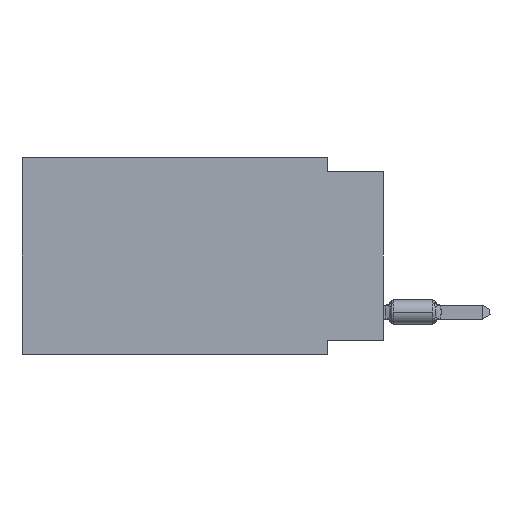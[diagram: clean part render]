
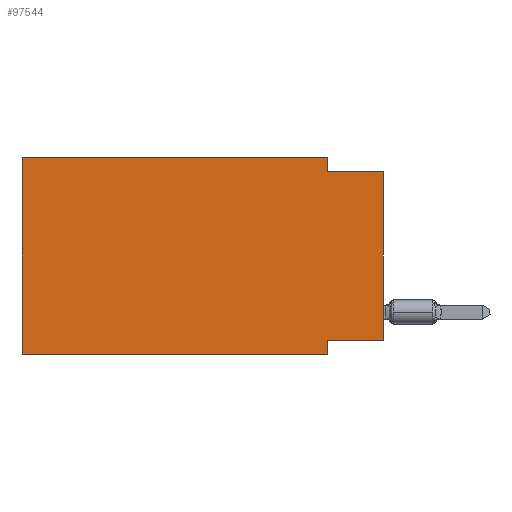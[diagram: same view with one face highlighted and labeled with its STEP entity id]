
A CAD part, left-side view. The second image highlights one B-rep face of the part: STEP entity #97544.
In plain terms, the highlighted planar face has unit normal (-1, 0, 0).
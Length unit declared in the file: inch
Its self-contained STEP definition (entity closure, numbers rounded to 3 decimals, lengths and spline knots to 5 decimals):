
#683 = PLANE ( 'NONE',  #84745 ) ;
#5026 = DIRECTION ( 'NONE',  ( 0., -1., 0. ) ) ;
#6773 = EDGE_CURVE ( 'NONE', #51343, #54908, #22327, .T. ) ;
#7010 = CARTESIAN_POINT ( 'NONE',  ( 0., 0.645, 0. ) ) ;
#9215 = VECTOR ( 'NONE', #25521, 39.37008 ) ;
#12195 = VERTEX_POINT ( 'NONE', #44199 ) ;
#14014 = CARTESIAN_POINT ( 'NONE',  ( 0., 0., -0.325 ) ) ;
#14069 = CARTESIAN_POINT ( 'NONE',  ( 0., 0.1, -0.325 ) ) ;
#15160 = FACE_OUTER_BOUND ( 'NONE', #84320, .T. ) ;
#15401 = LINE ( 'NONE', #47994, #83148 ) ;
#16739 = DIRECTION ( 'NONE',  ( 0., 0., 1. ) ) ;
#20035 = LINE ( 'NONE', #54736, #75508 ) ;
#21711 = CARTESIAN_POINT ( 'NONE',  ( 0., 0.1, -0.025 ) ) ;
#21777 = EDGE_CURVE ( 'NONE', #70939, #39694, #88263, .T. ) ;
#22327 = LINE ( 'NONE', #91770, #9215 ) ;
#23182 = DIRECTION ( 'NONE',  ( 0., 0., -1. ) ) ;
#24846 = ORIENTED_EDGE ( 'NONE', *, *, #70834, .T. ) ;
#25521 = DIRECTION ( 'NONE',  ( 0., -1., 0. ) ) ;
#28022 = CARTESIAN_POINT ( 'NONE',  ( 0., 0.1, 0. ) ) ;
#29117 = VECTOR ( 'NONE', #37099, 39.37008 ) ;
#32176 = DIRECTION ( 'NONE',  ( 0., 1., 0. ) ) ;
#33823 = DIRECTION ( 'NONE',  ( 1., 0., 0. ) ) ;
#34258 = LINE ( 'NONE', #73814, #103208 ) ;
#37099 = DIRECTION ( 'NONE',  ( 0., 0., -1. ) ) ;
#37621 = CARTESIAN_POINT ( 'NONE',  ( 0., 0.1, 0. ) ) ;
#39694 = VERTEX_POINT ( 'NONE', #7010 ) ;
#41822 = CARTESIAN_POINT ( 'NONE',  ( 0., 0.645, -0.35 ) ) ;
#44199 = CARTESIAN_POINT ( 'NONE',  ( 0., 0.1, -0.35 ) ) ;
#44645 = EDGE_CURVE ( 'NONE', #47113, #51343, #45103, .T. ) ;
#45103 = LINE ( 'NONE', #28022, #29117 ) ;
#46551 = DIRECTION ( 'NONE',  ( 0., 0., 1. ) ) ;
#47089 = EDGE_CURVE ( 'NONE', #70939, #12195, #20035, .T. ) ;
#47113 = VERTEX_POINT ( 'NONE', #37621 ) ;
#47994 = CARTESIAN_POINT ( 'NONE',  ( 0., 0.645, 0. ) ) ;
#49284 = ORIENTED_EDGE ( 'NONE', *, *, #6773, .F. ) ;
#50592 = ORIENTED_EDGE ( 'NONE', *, *, #21777, .F. ) ;
#50733 = VECTOR ( 'NONE', #23182, 39.37008 ) ;
#51343 = VERTEX_POINT ( 'NONE', #21711 ) ;
#54736 = CARTESIAN_POINT ( 'NONE',  ( 0., 0.645, -0.35 ) ) ;
#54908 = VERTEX_POINT ( 'NONE', #104508 ) ;
#55809 = CARTESIAN_POINT ( 'NONE',  ( 0., 0.1, -0.35 ) ) ;
#56295 = LINE ( 'NONE', #89950, #70344 ) ;
#56703 = CARTESIAN_POINT ( 'NONE',  ( 0., 0.645, 0. ) ) ;
#60435 = VERTEX_POINT ( 'NONE', #14069 ) ;
#66154 = DIRECTION ( 'NONE',  ( 0., -1., 0. ) ) ;
#69781 = VECTOR ( 'NONE', #46551, 39.37008 ) ;
#70344 = VECTOR ( 'NONE', #16739, 39.37008 ) ;
#70834 = EDGE_CURVE ( 'NONE', #75161, #54908, #56295, .T. ) ;
#70938 = ORIENTED_EDGE ( 'NONE', *, *, #82211, .F. ) ;
#70939 = VERTEX_POINT ( 'NONE', #41822 ) ;
#72389 = ORIENTED_EDGE ( 'NONE', *, *, #84184, .F. ) ;
#73814 = CARTESIAN_POINT ( 'NONE',  ( 0., 0., -0.325 ) ) ;
#75161 = VERTEX_POINT ( 'NONE', #14014 ) ;
#75508 = VECTOR ( 'NONE', #5026, 39.37008 ) ;
#76800 = ORIENTED_EDGE ( 'NONE', *, *, #47089, .T. ) ;
#77573 = ORIENTED_EDGE ( 'NONE', *, *, #44645, .F. ) ;
#82211 = EDGE_CURVE ( 'NONE', #39694, #47113, #15401, .T. ) ;
#83148 = VECTOR ( 'NONE', #66154, 39.37008 ) ;
#83216 = ORIENTED_EDGE ( 'NONE', *, *, #95433, .F. ) ;
#84184 = EDGE_CURVE ( 'NONE', #60435, #12195, #87294, .T. ) ;
#84320 = EDGE_LOOP ( 'NONE', ( #24846, #49284, #77573, #70938, #50592, #76800, #72389, #83216 ) ) ;
#84745 = AXIS2_PLACEMENT_3D ( 'NONE', #98525, #33823, #104936 ) ;
#87294 = LINE ( 'NONE', #55809, #50733 ) ;
#88263 = LINE ( 'NONE', #56703, #69781 ) ;
#89950 = CARTESIAN_POINT ( 'NONE',  ( 0., 0., 0. ) ) ;
#91770 = CARTESIAN_POINT ( 'NONE',  ( 0., 0., -0.025 ) ) ;
#95433 = EDGE_CURVE ( 'NONE', #75161, #60435, #34258, .T. ) ;
#97544 = ADVANCED_FACE ( 'NONE', ( #15160 ), #683, .F. ) ;
#98525 = CARTESIAN_POINT ( 'NONE',  ( 0., 0.645, 0. ) ) ;
#103208 = VECTOR ( 'NONE', #32176, 39.37008 ) ;
#104508 = CARTESIAN_POINT ( 'NONE',  ( 0., 0., -0.025 ) ) ;
#104936 = DIRECTION ( 'NONE',  ( 0., 0., -1. ) ) ;
